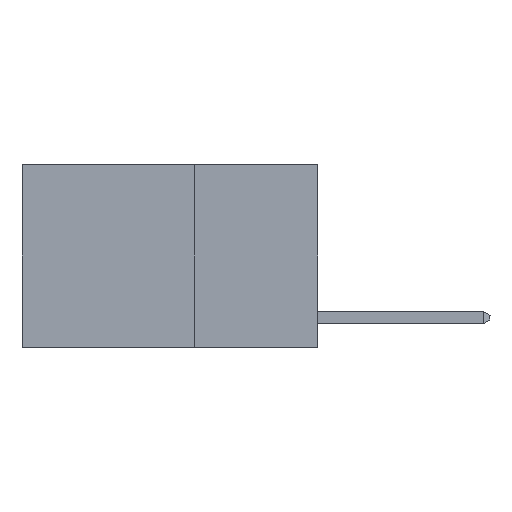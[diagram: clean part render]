
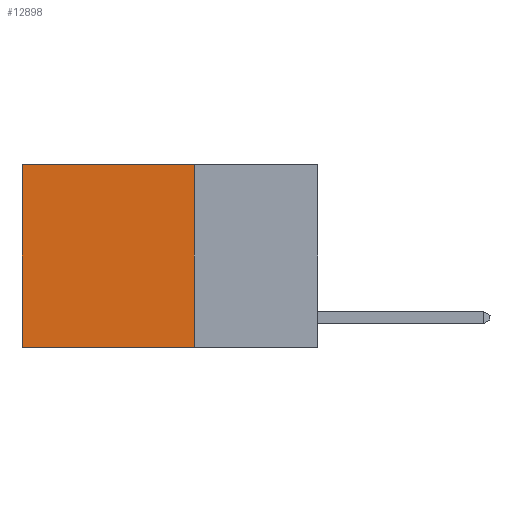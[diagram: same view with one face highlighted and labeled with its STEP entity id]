
A CAD part, left-side view. The second image highlights one B-rep face of the part: STEP entity #12898.
In plain terms, the highlighted planar face has unit normal (-1, 0, 0).
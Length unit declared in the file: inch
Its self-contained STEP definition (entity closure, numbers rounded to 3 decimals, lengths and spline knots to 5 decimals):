
#271 = VECTOR ( 'NONE', #2255, 39.37008 ) ;
#533 = DIRECTION ( 'NONE',  ( 0., 1., 0. ) ) ;
#1074 = CARTESIAN_POINT ( 'NONE',  ( 0.2625, 0.25, 0. ) ) ;
#1155 = AXIS2_PLACEMENT_3D ( 'NONE', #1074, #5161, #3176 ) ;
#1191 = CARTESIAN_POINT ( 'NONE',  ( 0.2625, 0.6, 0. ) ) ;
#1598 = ORIENTED_EDGE ( 'NONE', *, *, #5878, .F. ) ;
#2233 = VERTEX_POINT ( 'NONE', #1191 ) ;
#2255 = DIRECTION ( 'NONE',  ( 0., 1., 0. ) ) ;
#2309 = CARTESIAN_POINT ( 'NONE',  ( 0.2625, 0.25, -0.37 ) ) ;
#2557 = ORIENTED_EDGE ( 'NONE', *, *, #11434, .F. ) ;
#3074 = CARTESIAN_POINT ( 'NONE',  ( 0.2625, 0.25, -0.37 ) ) ;
#3176 = DIRECTION ( 'NONE',  ( 0., 0., -1. ) ) ;
#3340 = CARTESIAN_POINT ( 'NONE',  ( 0.2625, 0.6, 0. ) ) ;
#3479 = CARTESIAN_POINT ( 'NONE',  ( 0.2625, 0.6, -0.37 ) ) ;
#4033 = CARTESIAN_POINT ( 'NONE',  ( 0.2625, 0.25, 0. ) ) ;
#4186 = VECTOR ( 'NONE', #533, 39.37008 ) ;
#4600 = DIRECTION ( 'NONE',  ( 0., 0., -1. ) ) ;
#4666 = EDGE_CURVE ( 'NONE', #2233, #7222, #6637, .T. ) ;
#5161 = DIRECTION ( 'NONE',  ( 1., 0., 0. ) ) ;
#5645 = LINE ( 'NONE', #9796, #4186 ) ;
#5757 = EDGE_LOOP ( 'NONE', ( #10856, #1598, #2557, #10645 ) ) ;
#5878 = EDGE_CURVE ( 'NONE', #7598, #7222, #12534, .T. ) ;
#5913 = CARTESIAN_POINT ( 'NONE',  ( 0.2625, 0.25, 0. ) ) ;
#6195 = PLANE ( 'NONE',  #1155 ) ;
#6637 = LINE ( 'NONE', #3340, #6969 ) ;
#6969 = VECTOR ( 'NONE', #4600, 39.37008 ) ;
#7222 = VERTEX_POINT ( 'NONE', #3479 ) ;
#7598 = VERTEX_POINT ( 'NONE', #2309 ) ;
#8776 = DIRECTION ( 'NONE',  ( 0., 0., -1. ) ) ;
#9796 = CARTESIAN_POINT ( 'NONE',  ( 0.2625, 0.25, 0. ) ) ;
#10015 = VECTOR ( 'NONE', #8776, 39.37008 ) ;
#10109 = EDGE_CURVE ( 'NONE', #13179, #2233, #5645, .T. ) ;
#10645 = ORIENTED_EDGE ( 'NONE', *, *, #10109, .T. ) ;
#10856 = ORIENTED_EDGE ( 'NONE', *, *, #4666, .T. ) ;
#11381 = FACE_OUTER_BOUND ( 'NONE', #5757, .T. ) ;
#11434 = EDGE_CURVE ( 'NONE', #13179, #7598, #13067, .T. ) ;
#12534 = LINE ( 'NONE', #3074, #271 ) ;
#12898 = ADVANCED_FACE ( 'NONE', ( #11381 ), #6195, .F. ) ;
#13067 = LINE ( 'NONE', #5913, #10015 ) ;
#13179 = VERTEX_POINT ( 'NONE', #4033 ) ;
